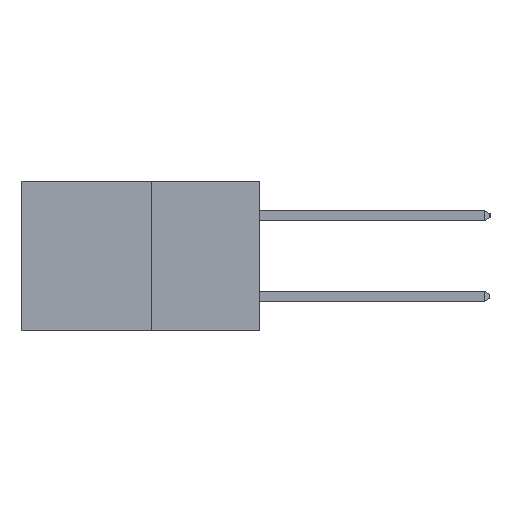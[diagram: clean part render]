
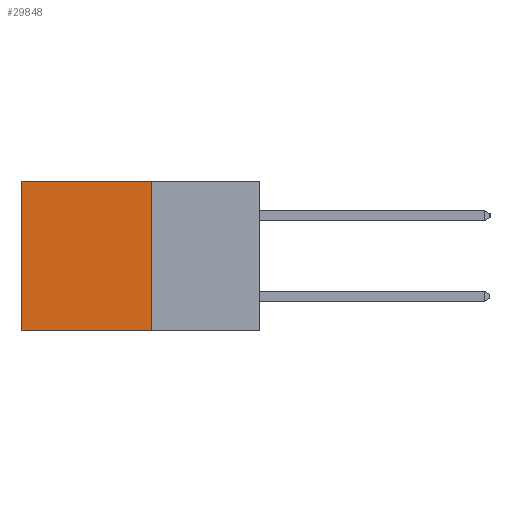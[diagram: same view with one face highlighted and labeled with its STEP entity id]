
A CAD part, left-side view. The second image highlights one B-rep face of the part: STEP entity #29848.
In plain terms, the highlighted planar face has unit normal (-1, 0, 0).
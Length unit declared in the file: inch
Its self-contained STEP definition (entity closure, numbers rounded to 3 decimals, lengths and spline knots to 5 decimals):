
#342 = FACE_OUTER_BOUND ( 'NONE', #4801, .T. ) ;
#610 = CARTESIAN_POINT ( 'NONE',  ( 0.277, 0.59, -0.37 ) ) ;
#3632 = EDGE_CURVE ( 'NONE', #28746, #17946, #29417, .T. ) ;
#3871 = VECTOR ( 'NONE', #17751, 39.37008 ) ;
#4183 = VECTOR ( 'NONE', #12553, 39.37008 ) ;
#4801 = EDGE_LOOP ( 'NONE', ( #22099, #15636, #14917, #7751 ) ) ;
#5113 = AXIS2_PLACEMENT_3D ( 'NONE', #10158, #26548, #12543 ) ;
#5823 = CARTESIAN_POINT ( 'NONE',  ( 0.277, 0.59, 0. ) ) ;
#6253 = EDGE_CURVE ( 'NONE', #15585, #28746, #10064, .T. ) ;
#7751 = ORIENTED_EDGE ( 'NONE', *, *, #18530, .T. ) ;
#9723 = CARTESIAN_POINT ( 'NONE',  ( 0.277, 0.27, -0.37 ) ) ;
#9997 = DIRECTION ( 'NONE',  ( 0., 1., 0. ) ) ;
#10064 = LINE ( 'NONE', #10608, #3871 ) ;
#10158 = CARTESIAN_POINT ( 'NONE',  ( 0.277, 0.27, -0.37 ) ) ;
#10383 = LINE ( 'NONE', #28873, #4183 ) ;
#10501 = VECTOR ( 'NONE', #21382, 39.37008 ) ;
#10608 = CARTESIAN_POINT ( 'NONE',  ( 0.277, 0.27, -0.37 ) ) ;
#11530 = VERTEX_POINT ( 'NONE', #5823 ) ;
#11534 = VECTOR ( 'NONE', #9997, 39.37008 ) ;
#12543 = DIRECTION ( 'NONE',  ( 0., 0., -1. ) ) ;
#12553 = DIRECTION ( 'NONE',  ( 0., 0., -1. ) ) ;
#12583 = CARTESIAN_POINT ( 'NONE',  ( 0.277, 0.27, -0.37 ) ) ;
#14283 = CARTESIAN_POINT ( 'NONE',  ( 0.277, 0.27, 0. ) ) ;
#14917 = ORIENTED_EDGE ( 'NONE', *, *, #6253, .F. ) ;
#15585 = VERTEX_POINT ( 'NONE', #20108 ) ;
#15636 = ORIENTED_EDGE ( 'NONE', *, *, #3632, .F. ) ;
#17751 = DIRECTION ( 'NONE',  ( 0., 0., -1. ) ) ;
#17946 = VERTEX_POINT ( 'NONE', #610 ) ;
#18530 = EDGE_CURVE ( 'NONE', #15585, #11530, #29147, .T. ) ;
#20108 = CARTESIAN_POINT ( 'NONE',  ( 0.277, 0.27, 0. ) ) ;
#21382 = DIRECTION ( 'NONE',  ( 0., 1., 0. ) ) ;
#22099 = ORIENTED_EDGE ( 'NONE', *, *, #27318, .T. ) ;
#24241 = PLANE ( 'NONE',  #5113 ) ;
#26548 = DIRECTION ( 'NONE',  ( 1., 0., 0. ) ) ;
#27318 = EDGE_CURVE ( 'NONE', #11530, #17946, #10383, .T. ) ;
#28746 = VERTEX_POINT ( 'NONE', #12583 ) ;
#28873 = CARTESIAN_POINT ( 'NONE',  ( 0.277, 0.59, -0.37 ) ) ;
#29147 = LINE ( 'NONE', #14283, #10501 ) ;
#29417 = LINE ( 'NONE', #9723, #11534 ) ;
#29848 = ADVANCED_FACE ( 'NONE', ( #342 ), #24241, .F. ) ;
